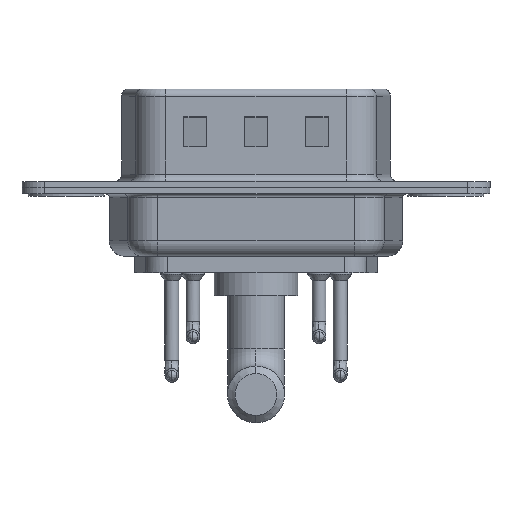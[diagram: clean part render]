
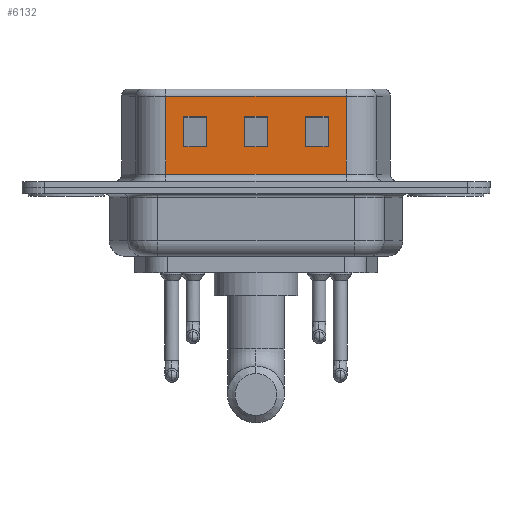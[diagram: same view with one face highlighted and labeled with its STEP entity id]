
A CAD part, front view. The second image highlights one B-rep face of the part: STEP entity #6132.
In plain terms, the highlighted planar face has unit normal (0, -1, 0).
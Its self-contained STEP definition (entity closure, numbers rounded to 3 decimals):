
#52 = DIRECTION ( 'NONE',  ( 0., 0., -1. ) ) ;
#151 = VECTOR ( 'NONE', #9205, 1000. ) ;
#191 = EDGE_CURVE ( 'NONE', #6079, #10135, #15455, .T. ) ;
#512 = VECTOR ( 'NONE', #10080, 1000. ) ;
#514 = LINE ( 'NONE', #4315, #4997 ) ;
#615 = CARTESIAN_POINT ( 'NONE',  ( 15.75, -4.55, 4.705 ) ) ;
#1046 = VERTEX_POINT ( 'NONE', #12725 ) ;
#1086 = VECTOR ( 'NONE', #52, 1000. ) ;
#1119 = LINE ( 'NONE', #17430, #7510 ) ;
#1271 = AXIS2_PLACEMENT_3D ( 'NONE', #2725, #12400, #1302 ) ;
#1302 = DIRECTION ( 'NONE',  ( -1., 0., 0. ) ) ;
#1324 = VERTEX_POINT ( 'NONE', #5481 ) ;
#1510 = ORIENTED_EDGE ( 'NONE', *, *, #13062, .T. ) ;
#1947 = ORIENTED_EDGE ( 'NONE', *, *, #10308, .T. ) ;
#2507 = ORIENTED_EDGE ( 'NONE', *, *, #14778, .T. ) ;
#2548 = LINE ( 'NONE', #4041, #1086 ) ;
#2703 = LINE ( 'NONE', #13700, #4101 ) ;
#2725 = CARTESIAN_POINT ( 'NONE',  ( 18.451, -4.55, 6.52 ) ) ;
#2754 = VERTEX_POINT ( 'NONE', #2917 ) ;
#2811 = FACE_BOUND ( 'NONE', #9467, .T. ) ;
#2888 = FACE_OUTER_BOUND ( 'NONE', #3696, .T. ) ;
#2917 = CARTESIAN_POINT ( 'NONE',  ( 6.549, -4.55, 0.9 ) ) ;
#2948 = ORIENTED_EDGE ( 'NONE', *, *, #12472, .T. ) ;
#2999 = DIRECTION ( 'NONE',  ( 0., 0., 1. ) ) ;
#3038 = LINE ( 'NONE', #9707, #9474 ) ;
#3039 = DIRECTION ( 'NONE',  ( 0., 0., 1. ) ) ;
#3397 = CARTESIAN_POINT ( 'NONE',  ( 7.75, -4.55, 6.52 ) ) ;
#3696 = EDGE_LOOP ( 'NONE', ( #15426, #16084, #13628, #16349 ) ) ;
#3874 = CARTESIAN_POINT ( 'NONE',  ( 11.75, -4.55, 4.705 ) ) ;
#3924 = DIRECTION ( 'NONE',  ( 0., 0., -1. ) ) ;
#4041 = CARTESIAN_POINT ( 'NONE',  ( 9.25, -4.55, 6.52 ) ) ;
#4101 = VECTOR ( 'NONE', #5269, 1000. ) ;
#4186 = VERTEX_POINT ( 'NONE', #615 ) ;
#4315 = CARTESIAN_POINT ( 'NONE',  ( 22.451, -4.55, 2.705 ) ) ;
#4408 = DIRECTION ( 'NONE',  ( -1., 0., 0. ) ) ;
#4537 = ORIENTED_EDGE ( 'NONE', *, *, #16508, .T. ) ;
#4903 = EDGE_LOOP ( 'NONE', ( #17188, #8785, #2948, #9145 ) ) ;
#4997 = VECTOR ( 'NONE', #4408, 1000. ) ;
#5085 = LINE ( 'NONE', #14563, #14647 ) ;
#5191 = CARTESIAN_POINT ( 'NONE',  ( 18.451, -4.55, 4.705 ) ) ;
#5238 = VERTEX_POINT ( 'NONE', #5266 ) ;
#5266 = CARTESIAN_POINT ( 'NONE',  ( 17.25, -4.55, 4.705 ) ) ;
#5269 = DIRECTION ( 'NONE',  ( 1., 0., 0. ) ) ;
#5331 = ORIENTED_EDGE ( 'NONE', *, *, #13368, .T. ) ;
#5377 = FACE_BOUND ( 'NONE', #4903, .T. ) ;
#5481 = CARTESIAN_POINT ( 'NONE',  ( 7.75, -4.55, 4.705 ) ) ;
#5556 = CARTESIAN_POINT ( 'NONE',  ( 14.451, -4.55, 2.705 ) ) ;
#6079 = VERTEX_POINT ( 'NONE', #8308 ) ;
#6132 = ADVANCED_FACE ( 'NONE', ( #2811, #5377, #14872, #2888 ), #16210, .F. ) ;
#6321 = CARTESIAN_POINT ( 'NONE',  ( 18.451, -4.55, 6.02 ) ) ;
#6684 = EDGE_CURVE ( 'NONE', #2754, #15551, #2703, .T. ) ;
#6911 = VECTOR ( 'NONE', #2999, 1000. ) ;
#7235 = CARTESIAN_POINT ( 'NONE',  ( 18.451, -4.55, 6.02 ) ) ;
#7434 = EDGE_CURVE ( 'NONE', #4186, #5238, #14441, .T. ) ;
#7471 = VERTEX_POINT ( 'NONE', #3874 ) ;
#7510 = VECTOR ( 'NONE', #17268, 1000. ) ;
#7690 = EDGE_CURVE ( 'NONE', #16742, #16926, #12667, .T. ) ;
#8169 = DIRECTION ( 'NONE',  ( -1., 0., 0. ) ) ;
#8308 = CARTESIAN_POINT ( 'NONE',  ( 13.25, -4.55, 2.705 ) ) ;
#8413 = ORIENTED_EDGE ( 'NONE', *, *, #12480, .T. ) ;
#8513 = CARTESIAN_POINT ( 'NONE',  ( 6.549, -4.55, 6.52 ) ) ;
#8729 = CARTESIAN_POINT ( 'NONE',  ( 18.451, -4.55, 2.705 ) ) ;
#8785 = ORIENTED_EDGE ( 'NONE', *, *, #13088, .T. ) ;
#9017 = VERTEX_POINT ( 'NONE', #13615 ) ;
#9122 = CARTESIAN_POINT ( 'NONE',  ( 22.451, -4.55, 4.705 ) ) ;
#9145 = ORIENTED_EDGE ( 'NONE', *, *, #7434, .T. ) ;
#9205 = DIRECTION ( 'NONE',  ( 1., 0., 0. ) ) ;
#9467 = EDGE_LOOP ( 'NONE', ( #2507, #1510, #8413, #5331 ) ) ;
#9474 = VECTOR ( 'NONE', #15198, 1000. ) ;
#9631 = DIRECTION ( 'NONE',  ( 1., 0., 0. ) ) ;
#9707 = CARTESIAN_POINT ( 'NONE',  ( 17.25, -4.55, 6.52 ) ) ;
#9839 = LINE ( 'NONE', #8513, #15364 ) ;
#9924 = CARTESIAN_POINT ( 'NONE',  ( 9.25, -4.55, 4.705 ) ) ;
#10014 = EDGE_CURVE ( 'NONE', #16926, #2754, #9839, .T. ) ;
#10080 = DIRECTION ( 'NONE',  ( -1., 0., 0. ) ) ;
#10114 = LINE ( 'NONE', #14110, #6911 ) ;
#10135 = VERTEX_POINT ( 'NONE', #12937 ) ;
#10196 = EDGE_CURVE ( 'NONE', #5238, #1046, #3038, .T. ) ;
#10308 = EDGE_CURVE ( 'NONE', #7471, #15972, #15022, .T. ) ;
#10508 = VECTOR ( 'NONE', #11210, 1000. ) ;
#10649 = LINE ( 'NONE', #5556, #16605 ) ;
#10656 = CARTESIAN_POINT ( 'NONE',  ( 18.451, -4.55, 0.9 ) ) ;
#11210 = DIRECTION ( 'NONE',  ( 1., 0., 0. ) ) ;
#11318 = CARTESIAN_POINT ( 'NONE',  ( 15.75, -4.55, 6.52 ) ) ;
#11480 = LINE ( 'NONE', #11318, #14084 ) ;
#11485 = VERTEX_POINT ( 'NONE', #12526 ) ;
#12400 = DIRECTION ( 'NONE',  ( 0., 1., 0. ) ) ;
#12472 = EDGE_CURVE ( 'NONE', #16018, #4186, #11480, .T. ) ;
#12480 = EDGE_CURVE ( 'NONE', #9017, #1324, #16888, .T. ) ;
#12526 = CARTESIAN_POINT ( 'NONE',  ( 9.25, -4.55, 2.705 ) ) ;
#12578 = ORIENTED_EDGE ( 'NONE', *, *, #191, .T. ) ;
#12667 = LINE ( 'NONE', #7235, #512 ) ;
#12725 = CARTESIAN_POINT ( 'NONE',  ( 17.25, -4.55, 2.705 ) ) ;
#12937 = CARTESIAN_POINT ( 'NONE',  ( 11.75, -4.55, 2.705 ) ) ;
#13062 = EDGE_CURVE ( 'NONE', #11485, #9017, #10649, .T. ) ;
#13088 = EDGE_CURVE ( 'NONE', #1046, #16018, #514, .T. ) ;
#13368 = EDGE_CURVE ( 'NONE', #1324, #17536, #13879, .T. ) ;
#13615 = CARTESIAN_POINT ( 'NONE',  ( 7.75, -4.55, 2.705 ) ) ;
#13621 = CARTESIAN_POINT ( 'NONE',  ( 14.451, -4.55, 4.705 ) ) ;
#13628 = ORIENTED_EDGE ( 'NONE', *, *, #10014, .T. ) ;
#13630 = EDGE_CURVE ( 'NONE', #16742, #15551, #5085, .T. ) ;
#13700 = CARTESIAN_POINT ( 'NONE',  ( 18.451, -4.55, 0.9 ) ) ;
#13772 = ORIENTED_EDGE ( 'NONE', *, *, #15738, .T. ) ;
#13879 = LINE ( 'NONE', #13621, #16915 ) ;
#14084 = VECTOR ( 'NONE', #3039, 1000. ) ;
#14110 = CARTESIAN_POINT ( 'NONE',  ( 11.75, -4.55, 6.52 ) ) ;
#14203 = EDGE_LOOP ( 'NONE', ( #1947, #4537, #12578, #13772 ) ) ;
#14441 = LINE ( 'NONE', #9122, #151 ) ;
#14563 = CARTESIAN_POINT ( 'NONE',  ( 18.451, -4.55, 6.52 ) ) ;
#14647 = VECTOR ( 'NONE', #3924, 1000. ) ;
#14778 = EDGE_CURVE ( 'NONE', #17536, #11485, #2548, .T. ) ;
#14872 = FACE_BOUND ( 'NONE', #14203, .T. ) ;
#15022 = LINE ( 'NONE', #5191, #10508 ) ;
#15198 = DIRECTION ( 'NONE',  ( 0., 0., -1. ) ) ;
#15240 = DIRECTION ( 'NONE',  ( 0., 0., -1. ) ) ;
#15364 = VECTOR ( 'NONE', #15240, 1000. ) ;
#15375 = DIRECTION ( 'NONE',  ( 0., 0., 1. ) ) ;
#15426 = ORIENTED_EDGE ( 'NONE', *, *, #13630, .F. ) ;
#15455 = LINE ( 'NONE', #8729, #16849 ) ;
#15551 = VERTEX_POINT ( 'NONE', #10656 ) ;
#15738 = EDGE_CURVE ( 'NONE', #10135, #7471, #10114, .T. ) ;
#15972 = VERTEX_POINT ( 'NONE', #17451 ) ;
#16018 = VERTEX_POINT ( 'NONE', #17365 ) ;
#16084 = ORIENTED_EDGE ( 'NONE', *, *, #7690, .T. ) ;
#16210 = PLANE ( 'NONE',  #1271 ) ;
#16342 = VECTOR ( 'NONE', #15375, 1000. ) ;
#16349 = ORIENTED_EDGE ( 'NONE', *, *, #6684, .T. ) ;
#16508 = EDGE_CURVE ( 'NONE', #15972, #6079, #1119, .T. ) ;
#16605 = VECTOR ( 'NONE', #8169, 1000. ) ;
#16742 = VERTEX_POINT ( 'NONE', #6321 ) ;
#16849 = VECTOR ( 'NONE', #16971, 1000. ) ;
#16888 = LINE ( 'NONE', #3397, #16342 ) ;
#16915 = VECTOR ( 'NONE', #9631, 1000. ) ;
#16926 = VERTEX_POINT ( 'NONE', #17506 ) ;
#16971 = DIRECTION ( 'NONE',  ( -1., 0., 0. ) ) ;
#17188 = ORIENTED_EDGE ( 'NONE', *, *, #10196, .T. ) ;
#17268 = DIRECTION ( 'NONE',  ( 0., 0., -1. ) ) ;
#17365 = CARTESIAN_POINT ( 'NONE',  ( 15.75, -4.55, 2.705 ) ) ;
#17430 = CARTESIAN_POINT ( 'NONE',  ( 13.25, -4.55, 6.52 ) ) ;
#17451 = CARTESIAN_POINT ( 'NONE',  ( 13.25, -4.55, 4.705 ) ) ;
#17506 = CARTESIAN_POINT ( 'NONE',  ( 6.549, -4.55, 6.02 ) ) ;
#17536 = VERTEX_POINT ( 'NONE', #9924 ) ;
